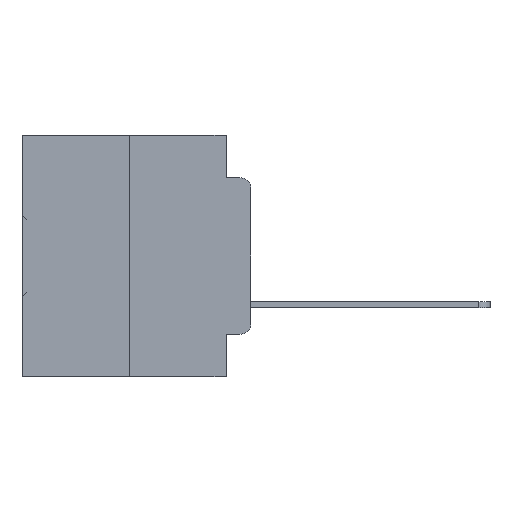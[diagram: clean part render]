
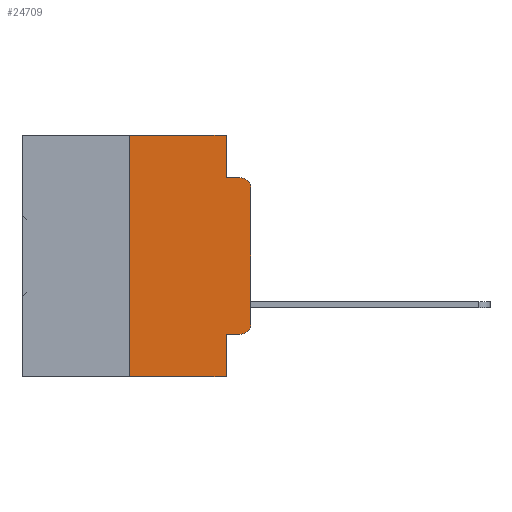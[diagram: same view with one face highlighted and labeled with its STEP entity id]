
A CAD part, left-side view. The second image highlights one B-rep face of the part: STEP entity #24709.
In plain terms, the highlighted planar face has unit normal (-1, 0, 0).
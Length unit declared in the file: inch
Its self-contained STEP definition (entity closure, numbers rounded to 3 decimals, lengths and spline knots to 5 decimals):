
#77 = DIRECTION ( 'NONE',  ( 0., 0., -1. ) ) ;
#201 = EDGE_CURVE ( 'NONE', #29052, #28850, #5348, .T. ) ;
#1168 = VERTEX_POINT ( 'NONE', #21369 ) ;
#1182 = VERTEX_POINT ( 'NONE', #26895 ) ;
#1465 = DIRECTION ( 'NONE',  ( 0., -1., 0. ) ) ;
#1738 = EDGE_CURVE ( 'NONE', #1182, #26139, #14785, .T. ) ;
#2211 = ORIENTED_EDGE ( 'NONE', *, *, #13559, .T. ) ;
#2709 = ORIENTED_EDGE ( 'NONE', *, *, #201, .T. ) ;
#2797 = EDGE_CURVE ( 'NONE', #34016, #1182, #17732, .T. ) ;
#2814 = CARTESIAN_POINT ( 'NONE',  ( 0., 0.051, -0.4115 ) ) ;
#3472 = DIRECTION ( 'NONE',  ( -1., 0., 0. ) ) ;
#4830 = CARTESIAN_POINT ( 'NONE',  ( 0., 0.051, -0.0885 ) ) ;
#4877 = VECTOR ( 'NONE', #25722, 39.37008 ) ;
#5245 = CARTESIAN_POINT ( 'NONE',  ( 0., 0.25, -0.5 ) ) ;
#5348 = LINE ( 'NONE', #14016, #27310 ) ;
#5679 = PLANE ( 'NONE',  #12640 ) ;
#6024 = CARTESIAN_POINT ( 'NONE',  ( 0., 0.051, -0.4115 ) ) ;
#6885 = LINE ( 'NONE', #33720, #27913 ) ;
#7288 = EDGE_CURVE ( 'NONE', #12133, #9267, #10848, .T. ) ;
#7337 = CARTESIAN_POINT ( 'NONE',  ( 0., 0.02, -0.4115 ) ) ;
#7765 = CARTESIAN_POINT ( 'NONE',  ( 0., 0.051, -0.5 ) ) ;
#8269 = VECTOR ( 'NONE', #32216, 39.37008 ) ;
#9090 = CIRCLE ( 'NONE', #14605, 0.02 ) ;
#9267 = VERTEX_POINT ( 'NONE', #7337 ) ;
#10848 = LINE ( 'NONE', #6024, #19064 ) ;
#11238 = CARTESIAN_POINT ( 'NONE',  ( 0., 0.473, 0. ) ) ;
#11546 = CARTESIAN_POINT ( 'NONE',  ( 0., 0.051, -0.0885 ) ) ;
#11587 = DIRECTION ( 'NONE',  ( 0., -1., 0. ) ) ;
#12062 = CARTESIAN_POINT ( 'NONE',  ( 0., 0.051, 0. ) ) ;
#12133 = VERTEX_POINT ( 'NONE', #2814 ) ;
#12640 = AXIS2_PLACEMENT_3D ( 'NONE', #11238, #16809, #77 ) ;
#12881 = EDGE_CURVE ( 'NONE', #23998, #1168, #13564, .T. ) ;
#13559 = EDGE_CURVE ( 'NONE', #9267, #29052, #33849, .T. ) ;
#13564 = LINE ( 'NONE', #11546, #27255 ) ;
#13662 = ORIENTED_EDGE ( 'NONE', *, *, #22754, .F. ) ;
#14016 = CARTESIAN_POINT ( 'NONE',  ( 0., 0., 0. ) ) ;
#14344 = DIRECTION ( 'NONE',  ( 0., -1., 0. ) ) ;
#14464 = CARTESIAN_POINT ( 'NONE',  ( 0., 0.02, -0.1085 ) ) ;
#14554 = FACE_OUTER_BOUND ( 'NONE', #29404, .T. ) ;
#14605 = AXIS2_PLACEMENT_3D ( 'NONE', #14464, #33423, #17234 ) ;
#14778 = DIRECTION ( 'NONE',  ( 0., 0., -1. ) ) ;
#14785 = LINE ( 'NONE', #23662, #22943 ) ;
#14955 = ORIENTED_EDGE ( 'NONE', *, *, #2797, .F. ) ;
#15619 = LINE ( 'NONE', #18744, #8269 ) ;
#16809 = DIRECTION ( 'NONE',  ( 1., 0., 0. ) ) ;
#17054 = ORIENTED_EDGE ( 'NONE', *, *, #12881, .F. ) ;
#17228 = DIRECTION ( 'NONE',  ( 0., 0., 1. ) ) ;
#17234 = DIRECTION ( 'NONE',  ( 0., 0., -1. ) ) ;
#17732 = LINE ( 'NONE', #25392, #30450 ) ;
#18744 = CARTESIAN_POINT ( 'NONE',  ( 0., 0.051, 0. ) ) ;
#19064 = VECTOR ( 'NONE', #11587, 39.37008 ) ;
#19588 = LINE ( 'NONE', #28388, #4877 ) ;
#20057 = CARTESIAN_POINT ( 'NONE',  ( 0., 0.02, -0.3915 ) ) ;
#21369 = CARTESIAN_POINT ( 'NONE',  ( 0., 0.02, -0.0885 ) ) ;
#22070 = EDGE_CURVE ( 'NONE', #28850, #1168, #9090, .T. ) ;
#22754 = EDGE_CURVE ( 'NONE', #26139, #23998, #6885, .T. ) ;
#22808 = DIRECTION ( 'NONE',  ( 0., 0., -1. ) ) ;
#22943 = VECTOR ( 'NONE', #1465, 39.37008 ) ;
#22983 = ORIENTED_EDGE ( 'NONE', *, *, #7288, .T. ) ;
#23541 = ORIENTED_EDGE ( 'NONE', *, *, #1738, .F. ) ;
#23662 = CARTESIAN_POINT ( 'NONE',  ( 0., 0.473, 0. ) ) ;
#23998 = VERTEX_POINT ( 'NONE', #4830 ) ;
#24005 = ORIENTED_EDGE ( 'NONE', *, *, #30102, .T. ) ;
#24109 = AXIS2_PLACEMENT_3D ( 'NONE', #20057, #3472, #22808 ) ;
#24709 = ADVANCED_FACE ( 'NONE', ( #14554 ), #5679, .F. ) ;
#25392 = CARTESIAN_POINT ( 'NONE',  ( 0., 0.25, 0. ) ) ;
#25722 = DIRECTION ( 'NONE',  ( 0., -1., 0. ) ) ;
#26035 = CARTESIAN_POINT ( 'NONE',  ( 0., 0., -0.3915 ) ) ;
#26139 = VERTEX_POINT ( 'NONE', #12062 ) ;
#26895 = CARTESIAN_POINT ( 'NONE',  ( 0., 0.25, 0. ) ) ;
#27255 = VECTOR ( 'NONE', #14344, 39.37008 ) ;
#27310 = VECTOR ( 'NONE', #32993, 39.37008 ) ;
#27913 = VECTOR ( 'NONE', #14778, 39.37008 ) ;
#28388 = CARTESIAN_POINT ( 'NONE',  ( 0., 0.473, -0.5 ) ) ;
#28850 = VERTEX_POINT ( 'NONE', #30464 ) ;
#29052 = VERTEX_POINT ( 'NONE', #26035 ) ;
#29404 = EDGE_LOOP ( 'NONE', ( #2709, #33548, #17054, #13662, #23541, #14955, #24005, #29887, #22983, #2211 ) ) ;
#29887 = ORIENTED_EDGE ( 'NONE', *, *, #32863, .F. ) ;
#30102 = EDGE_CURVE ( 'NONE', #34016, #32887, #19588, .T. ) ;
#30450 = VECTOR ( 'NONE', #17228, 39.37008 ) ;
#30464 = CARTESIAN_POINT ( 'NONE',  ( 0., 0., -0.1085 ) ) ;
#32216 = DIRECTION ( 'NONE',  ( 0., 0., -1. ) ) ;
#32863 = EDGE_CURVE ( 'NONE', #12133, #32887, #15619, .T. ) ;
#32887 = VERTEX_POINT ( 'NONE', #7765 ) ;
#32993 = DIRECTION ( 'NONE',  ( 0., 0., 1. ) ) ;
#33423 = DIRECTION ( 'NONE',  ( -1., 0., 0. ) ) ;
#33548 = ORIENTED_EDGE ( 'NONE', *, *, #22070, .T. ) ;
#33720 = CARTESIAN_POINT ( 'NONE',  ( 0., 0.051, 0. ) ) ;
#33849 = CIRCLE ( 'NONE', #24109, 0.02 ) ;
#34016 = VERTEX_POINT ( 'NONE', #5245 ) ;
